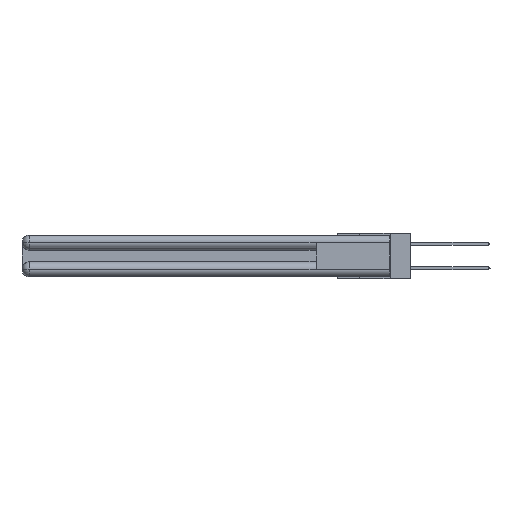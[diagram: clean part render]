
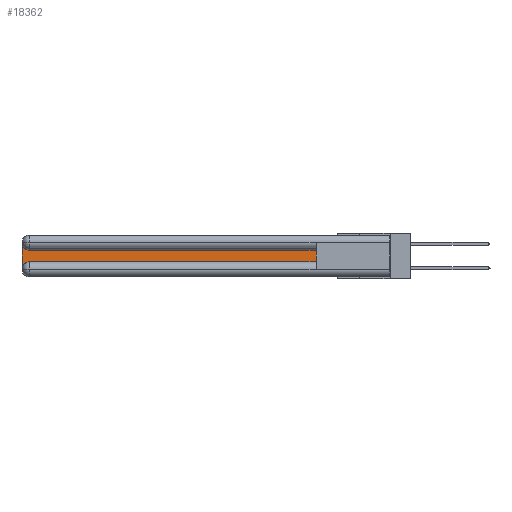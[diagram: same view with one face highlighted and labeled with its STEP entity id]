
A CAD part, left-side view. The second image highlights one B-rep face of the part: STEP entity #18362.
In plain terms, the highlighted planar face has unit normal (-1, 0, 0).
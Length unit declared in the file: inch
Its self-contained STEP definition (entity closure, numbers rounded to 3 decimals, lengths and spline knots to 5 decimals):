
#137 = CARTESIAN_POINT ( 'NONE',  ( 0.075, 2.94, -0.2775 ) ) ;
#1258 = ORIENTED_EDGE ( 'NONE', *, *, #25499, .T. ) ;
#2812 = DIRECTION ( 'NONE',  ( 1., 0., 0. ) ) ;
#3197 = AXIS2_PLACEMENT_3D ( 'NONE', #8240, #15989, #18980 ) ;
#5194 = CARTESIAN_POINT ( 'NONE',  ( 0.075, 3., -0.0625 ) ) ;
#5483 = FACE_OUTER_BOUND ( 'NONE', #18288, .T. ) ;
#6148 = VECTOR ( 'NONE', #9411, 39.37008 ) ;
#6270 = DIRECTION ( 'NONE',  ( 0., 0., 1. ) ) ;
#7898 = VERTEX_POINT ( 'NONE', #20524 ) ;
#8240 = CARTESIAN_POINT ( 'NONE',  ( 0.075, 2.94, -0.0625 ) ) ;
#9400 = LINE ( 'NONE', #31384, #23111 ) ;
#9411 = DIRECTION ( 'NONE',  ( 0., 1., 0. ) ) ;
#9445 = CIRCLE ( 'NONE', #3197, 0.06 ) ;
#10006 = CARTESIAN_POINT ( 'NONE',  ( 0.075, 3., -0.2775 ) ) ;
#10895 = EDGE_CURVE ( 'NONE', #27500, #16652, #28090, .T. ) ;
#10921 = DIRECTION ( 'NONE',  ( 0., 0., -1. ) ) ;
#13477 = CARTESIAN_POINT ( 'NONE',  ( 0.075, 3., -0.1225 ) ) ;
#14196 = CARTESIAN_POINT ( 'NONE',  ( 0.075, 2.94, -0.2175 ) ) ;
#15129 = DIRECTION ( 'NONE',  ( 0., -1., 0. ) ) ;
#15989 = DIRECTION ( 'NONE',  ( 1., 0., 0. ) ) ;
#16064 = CARTESIAN_POINT ( 'NONE',  ( 0.075, 3., -0.2175 ) ) ;
#16203 = VERTEX_POINT ( 'NONE', #5194 ) ;
#16636 = CARTESIAN_POINT ( 'NONE',  ( 0.075, 0.6, -0.1225 ) ) ;
#16652 = VERTEX_POINT ( 'NONE', #14196 ) ;
#16876 = CARTESIAN_POINT ( 'NONE',  ( 0.075, 2.94, -0.1225 ) ) ;
#16924 = ORIENTED_EDGE ( 'NONE', *, *, #21679, .T. ) ;
#17527 = EDGE_CURVE ( 'NONE', #16652, #7898, #9400, .T. ) ;
#18288 = EDGE_LOOP ( 'NONE', ( #16924, #31675, #33378, #18322, #20597, #1258 ) ) ;
#18322 = ORIENTED_EDGE ( 'NONE', *, *, #10895, .T. ) ;
#18362 = ADVANCED_FACE ( 'NONE', ( #5483 ), #27141, .F. ) ;
#18565 = LINE ( 'NONE', #33742, #6148 ) ;
#18980 = DIRECTION ( 'NONE',  ( 0., 0., -1. ) ) ;
#20524 = CARTESIAN_POINT ( 'NONE',  ( 0.075, 0.6, -0.2175 ) ) ;
#20597 = ORIENTED_EDGE ( 'NONE', *, *, #17527, .T. ) ;
#21679 = EDGE_CURVE ( 'NONE', #22063, #22051, #18565, .T. ) ;
#22051 = VERTEX_POINT ( 'NONE', #16876 ) ;
#22063 = VERTEX_POINT ( 'NONE', #16636 ) ;
#22495 = AXIS2_PLACEMENT_3D ( 'NONE', #13477, #2812, #29629 ) ;
#22558 = CARTESIAN_POINT ( 'NONE',  ( 0.075, 0.6, -0.2175 ) ) ;
#23111 = VECTOR ( 'NONE', #15129, 39.37008 ) ;
#23767 = AXIS2_PLACEMENT_3D ( 'NONE', #137, #27315, #10921 ) ;
#25499 = EDGE_CURVE ( 'NONE', #7898, #22063, #28526, .T. ) ;
#27141 = PLANE ( 'NONE',  #22495 ) ;
#27315 = DIRECTION ( 'NONE',  ( 1., 0., 0. ) ) ;
#27500 = VERTEX_POINT ( 'NONE', #10006 ) ;
#27659 = EDGE_CURVE ( 'NONE', #22051, #16203, #9445, .T. ) ;
#28090 = CIRCLE ( 'NONE', #23767, 0.06 ) ;
#28116 = VECTOR ( 'NONE', #29562, 39.37008 ) ;
#28526 = LINE ( 'NONE', #22558, #33163 ) ;
#29562 = DIRECTION ( 'NONE',  ( 0., 0., -1. ) ) ;
#29629 = DIRECTION ( 'NONE',  ( 0., 0., -1. ) ) ;
#29778 = LINE ( 'NONE', #16064, #28116 ) ;
#31384 = CARTESIAN_POINT ( 'NONE',  ( 0.075, 0.6, -0.2175 ) ) ;
#31675 = ORIENTED_EDGE ( 'NONE', *, *, #27659, .T. ) ;
#32820 = EDGE_CURVE ( 'NONE', #16203, #27500, #29778, .T. ) ;
#33163 = VECTOR ( 'NONE', #6270, 39.37008 ) ;
#33378 = ORIENTED_EDGE ( 'NONE', *, *, #32820, .T. ) ;
#33742 = CARTESIAN_POINT ( 'NONE',  ( 0.075, 0.6, -0.1225 ) ) ;
